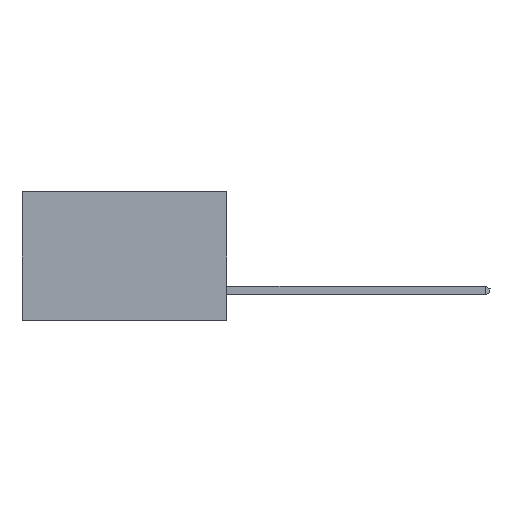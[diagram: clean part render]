
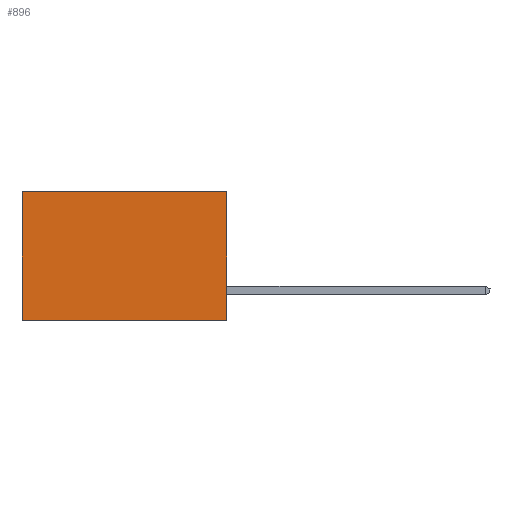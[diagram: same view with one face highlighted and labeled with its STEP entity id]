
A CAD part, left-side view. The second image highlights one B-rep face of the part: STEP entity #896.
In plain terms, the highlighted planar face has unit normal (-1, 0, 0).
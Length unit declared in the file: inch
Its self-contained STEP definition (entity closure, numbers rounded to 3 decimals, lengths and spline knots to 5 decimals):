
#489 = VECTOR ( 'NONE', #5003, 39.37008 ) ;
#840 = LINE ( 'NONE', #4118, #489 ) ;
#896 = ADVANCED_FACE ( 'NONE', ( #4277 ), #5110, .F. ) ;
#1331 = CARTESIAN_POINT ( 'NONE',  ( 0.277, 0., -0.37 ) ) ;
#1753 = EDGE_CURVE ( 'NONE', #9387, #6079, #5677, .T. ) ;
#2231 = LINE ( 'NONE', #6937, #9819 ) ;
#2303 = DIRECTION ( 'NONE',  ( 0., 1., 0. ) ) ;
#2428 = DIRECTION ( 'NONE',  ( 0., 0., -1. ) ) ;
#2433 = DIRECTION ( 'NONE',  ( 0., 0., -1. ) ) ;
#2455 = DIRECTION ( 'NONE',  ( 1., 0., 0. ) ) ;
#2711 = DIRECTION ( 'NONE',  ( 0., 1., 0. ) ) ;
#2725 = ORIENTED_EDGE ( 'NONE', *, *, #8110, .F. ) ;
#2767 = CARTESIAN_POINT ( 'NONE',  ( 0.277, 0., -0.37 ) ) ;
#2776 = VERTEX_POINT ( 'NONE', #9752 ) ;
#3460 = VECTOR ( 'NONE', #2433, 39.37008 ) ;
#3760 = EDGE_CURVE ( 'NONE', #2776, #9387, #2231, .T. ) ;
#4106 = CARTESIAN_POINT ( 'NONE',  ( 0.277, 0.59, 0. ) ) ;
#4118 = CARTESIAN_POINT ( 'NONE',  ( 0.277, 0., -0.37 ) ) ;
#4277 = FACE_OUTER_BOUND ( 'NONE', #8141, .T. ) ;
#4897 = ORIENTED_EDGE ( 'NONE', *, *, #3760, .T. ) ;
#5003 = DIRECTION ( 'NONE',  ( 0., 0., -1. ) ) ;
#5110 = PLANE ( 'NONE',  #8992 ) ;
#5613 = VECTOR ( 'NONE', #2303, 39.37008 ) ;
#5677 = LINE ( 'NONE', #9574, #3460 ) ;
#6079 = VERTEX_POINT ( 'NONE', #10009 ) ;
#6084 = EDGE_CURVE ( 'NONE', #7449, #6079, #7650, .T. ) ;
#6778 = ORIENTED_EDGE ( 'NONE', *, *, #1753, .T. ) ;
#6937 = CARTESIAN_POINT ( 'NONE',  ( 0.277, 0., 0. ) ) ;
#7449 = VERTEX_POINT ( 'NONE', #1331 ) ;
#7650 = LINE ( 'NONE', #9953, #5613 ) ;
#8110 = EDGE_CURVE ( 'NONE', #2776, #7449, #840, .T. ) ;
#8141 = EDGE_LOOP ( 'NONE', ( #6778, #8707, #2725, #4897 ) ) ;
#8707 = ORIENTED_EDGE ( 'NONE', *, *, #6084, .F. ) ;
#8992 = AXIS2_PLACEMENT_3D ( 'NONE', #2767, #2455, #2428 ) ;
#9387 = VERTEX_POINT ( 'NONE', #4106 ) ;
#9574 = CARTESIAN_POINT ( 'NONE',  ( 0.277, 0.59, -0.37 ) ) ;
#9752 = CARTESIAN_POINT ( 'NONE',  ( 0.277, 0., 0. ) ) ;
#9819 = VECTOR ( 'NONE', #2711, 39.37008 ) ;
#9953 = CARTESIAN_POINT ( 'NONE',  ( 0.277, 0., -0.37 ) ) ;
#10009 = CARTESIAN_POINT ( 'NONE',  ( 0.277, 0.59, -0.37 ) ) ;
